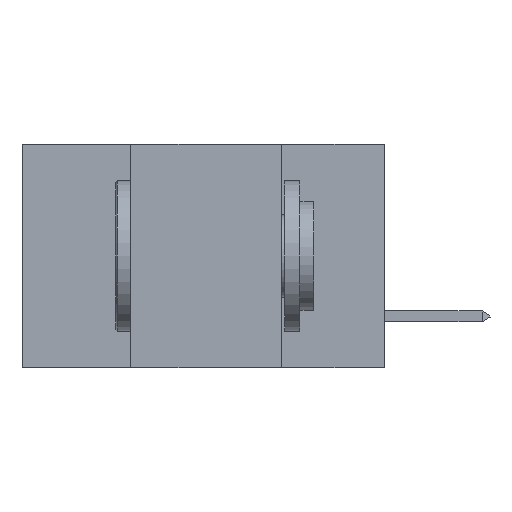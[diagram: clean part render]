
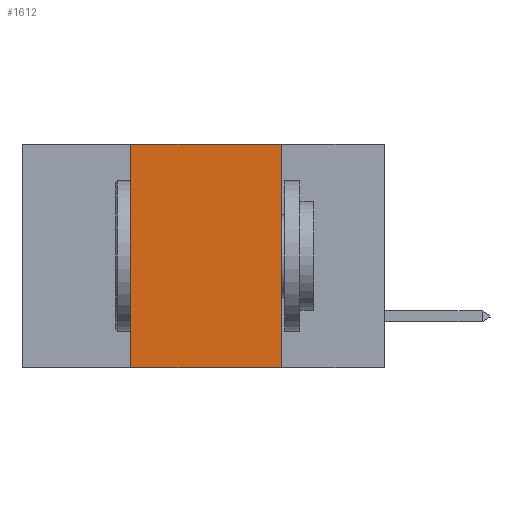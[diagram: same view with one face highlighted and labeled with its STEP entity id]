
A CAD part, left-side view. The second image highlights one B-rep face of the part: STEP entity #1612.
In plain terms, the highlighted planar face has unit normal (-1, 0, 0).
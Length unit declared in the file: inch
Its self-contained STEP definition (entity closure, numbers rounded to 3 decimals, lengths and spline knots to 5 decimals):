
#593 = CARTESIAN_POINT ( 'NONE',  ( 0., 0.17, 0. ) ) ;
#1586 = CARTESIAN_POINT ( 'NONE',  ( 0., 0.42, -0.37 ) ) ;
#1612 = ADVANCED_FACE ( 'NONE', ( #3586 ), #6567, .F. ) ;
#1936 = CARTESIAN_POINT ( 'NONE',  ( 0., 0.17, -0.37 ) ) ;
#1979 = VECTOR ( 'NONE', #6365, 39.37008 ) ;
#2029 = CARTESIAN_POINT ( 'NONE',  ( 0., 0.6, 0. ) ) ;
#2334 = DIRECTION ( 'NONE',  ( 0., 0., -1. ) ) ;
#2720 = DIRECTION ( 'NONE',  ( 0., 0., -1. ) ) ;
#2996 = LINE ( 'NONE', #3050, #1979 ) ;
#3050 = CARTESIAN_POINT ( 'NONE',  ( 0., 0.42, 0. ) ) ;
#3405 = VECTOR ( 'NONE', #7596, 39.37008 ) ;
#3457 = ORIENTED_EDGE ( 'NONE', *, *, #9627, .T. ) ;
#3533 = LINE ( 'NONE', #9809, #5125 ) ;
#3586 = FACE_OUTER_BOUND ( 'NONE', #5357, .T. ) ;
#3915 = DIRECTION ( 'NONE',  ( 1., 0., 0. ) ) ;
#4586 = AXIS2_PLACEMENT_3D ( 'NONE', #4703, #3915, #2334 ) ;
#4651 = ORIENTED_EDGE ( 'NONE', *, *, #7158, .F. ) ;
#4703 = CARTESIAN_POINT ( 'NONE',  ( 0., 0.6, 0. ) ) ;
#5125 = VECTOR ( 'NONE', #2720, 39.37008 ) ;
#5216 = LINE ( 'NONE', #8358, #6578 ) ;
#5357 = EDGE_LOOP ( 'NONE', ( #9491, #9784, #4651, #3457 ) ) ;
#5556 = VERTEX_POINT ( 'NONE', #6420 ) ;
#6365 = DIRECTION ( 'NONE',  ( 0., 0., 1. ) ) ;
#6420 = CARTESIAN_POINT ( 'NONE',  ( 0., 0.42, 0. ) ) ;
#6567 = PLANE ( 'NONE',  #4586 ) ;
#6575 = VERTEX_POINT ( 'NONE', #1586 ) ;
#6578 = VECTOR ( 'NONE', #9888, 39.37008 ) ;
#7101 = LINE ( 'NONE', #2029, #3405 ) ;
#7158 = EDGE_CURVE ( 'NONE', #6575, #5556, #2996, .T. ) ;
#7596 = DIRECTION ( 'NONE',  ( 0., -1., 0. ) ) ;
#8119 = VERTEX_POINT ( 'NONE', #1936 ) ;
#8209 = EDGE_CURVE ( 'NONE', #8396, #8119, #3533, .T. ) ;
#8358 = CARTESIAN_POINT ( 'NONE',  ( 0., 0.6, -0.37 ) ) ;
#8396 = VERTEX_POINT ( 'NONE', #593 ) ;
#8788 = EDGE_CURVE ( 'NONE', #5556, #8396, #7101, .T. ) ;
#9491 = ORIENTED_EDGE ( 'NONE', *, *, #8209, .F. ) ;
#9627 = EDGE_CURVE ( 'NONE', #6575, #8119, #5216, .T. ) ;
#9784 = ORIENTED_EDGE ( 'NONE', *, *, #8788, .F. ) ;
#9809 = CARTESIAN_POINT ( 'NONE',  ( 0., 0.17, 0. ) ) ;
#9888 = DIRECTION ( 'NONE',  ( 0., -1., 0. ) ) ;
